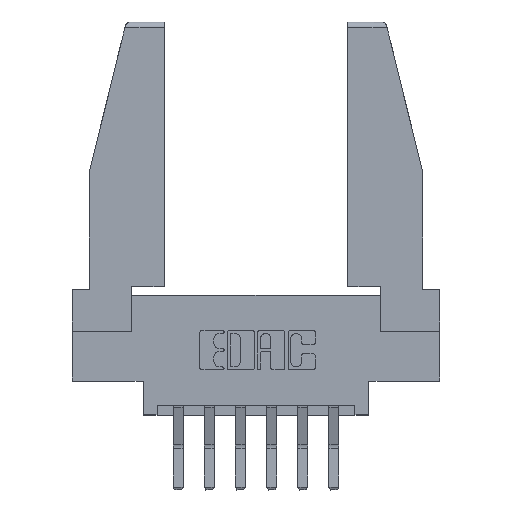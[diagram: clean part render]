
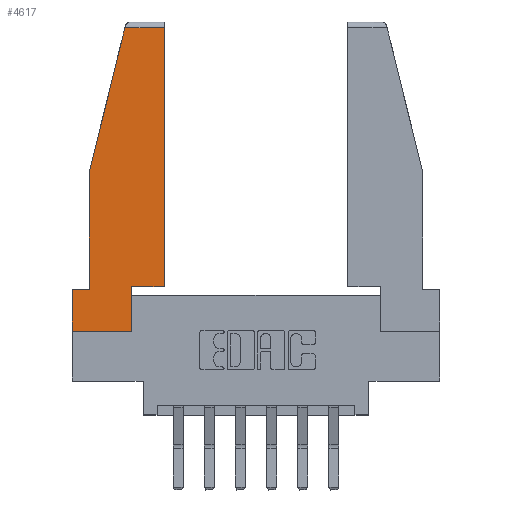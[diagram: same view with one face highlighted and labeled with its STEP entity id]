
A CAD part, top view. The second image highlights one B-rep face of the part: STEP entity #4617.
In plain terms, the highlighted planar face has unit normal (0, 0, 1).
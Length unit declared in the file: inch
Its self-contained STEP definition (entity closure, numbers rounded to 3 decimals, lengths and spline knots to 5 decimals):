
#335 = FACE_OUTER_BOUND ( 'NONE', #1896, .T. ) ;
#481 = ORIENTED_EDGE ( 'NONE', *, *, #3997, .T. ) ;
#562 = VERTEX_POINT ( 'NONE', #1322 ) ;
#895 = CARTESIAN_POINT ( 'NONE',  ( 0.461, 1.52, 0. ) ) ;
#1084 = VERTEX_POINT ( 'NONE', #895 ) ;
#1322 = CARTESIAN_POINT ( 'NONE',  ( 0.297, 0.223, 0. ) ) ;
#1429 = LINE ( 'NONE', #7265, #10963 ) ;
#1442 = CARTESIAN_POINT ( 'NONE',  ( 0.297, 0.223, 0. ) ) ;
#1462 = CARTESIAN_POINT ( 'NONE',  ( 0.086, 0.8, 0. ) ) ;
#1509 = VERTEX_POINT ( 'NONE', #9792 ) ;
#1642 = CARTESIAN_POINT ( 'NONE',  ( 0., 1.52, 0. ) ) ;
#1672 = VERTEX_POINT ( 'NONE', #10440 ) ;
#1715 = LINE ( 'NONE', #9343, #6177 ) ;
#1764 = DIRECTION ( 'NONE',  ( 0., 1., 0. ) ) ;
#1896 = EDGE_LOOP ( 'NONE', ( #10726, #5949, #8733, #7139, #9269, #3287, #5009, #481, #10562 ) ) ;
#2374 = VERTEX_POINT ( 'NONE', #8018 ) ;
#2620 = DIRECTION ( 'NONE',  ( 1., 0., 0. ) ) ;
#2673 = CARTESIAN_POINT ( 'NONE',  ( 0.086, 0.21, 0. ) ) ;
#2810 = CARTESIAN_POINT ( 'NONE',  ( 0.297, 0., 0. ) ) ;
#3060 = CARTESIAN_POINT ( 'NONE',  ( 0.2636, 1.52, 0. ) ) ;
#3287 = ORIENTED_EDGE ( 'NONE', *, *, #10573, .T. ) ;
#3321 = LINE ( 'NONE', #1642, #5349 ) ;
#3375 = CARTESIAN_POINT ( 'NONE',  ( 0.271, 1.55, 0. ) ) ;
#3633 = LINE ( 'NONE', #5037, #11858 ) ;
#3917 = DIRECTION ( 'NONE',  ( -1., 0., 0. ) ) ;
#3997 = EDGE_CURVE ( 'NONE', #1672, #562, #7844, .T. ) ;
#4175 = LINE ( 'NONE', #9431, #11834 ) ;
#4617 = ADVANCED_FACE ( 'NONE', ( #335 ), #5461, .T. ) ;
#5009 = ORIENTED_EDGE ( 'NONE', *, *, #9911, .T. ) ;
#5037 = CARTESIAN_POINT ( 'NONE',  ( 0.461, 0.223, 0. ) ) ;
#5315 = VECTOR ( 'NONE', #5523, 39.37008 ) ;
#5349 = VECTOR ( 'NONE', #7009, 39.37008 ) ;
#5395 = VECTOR ( 'NONE', #1764, 39.37008 ) ;
#5461 = PLANE ( 'NONE',  #7144 ) ;
#5523 = DIRECTION ( 'NONE',  ( 0., -1., 0. ) ) ;
#5735 = LINE ( 'NONE', #1442, #11045 ) ;
#5809 = VERTEX_POINT ( 'NONE', #1462 ) ;
#5937 = EDGE_CURVE ( 'NONE', #10702, #5809, #10527, .T. ) ;
#5949 = ORIENTED_EDGE ( 'NONE', *, *, #9807, .T. ) ;
#6177 = VECTOR ( 'NONE', #9271, 39.37008 ) ;
#6497 = CARTESIAN_POINT ( 'NONE',  ( 0., 0.21, 0. ) ) ;
#6789 = VERTEX_POINT ( 'NONE', #2673 ) ;
#6962 = EDGE_CURVE ( 'NONE', #5809, #6789, #8760, .T. ) ;
#7009 = DIRECTION ( 'NONE',  ( -1., 0., 0. ) ) ;
#7139 = ORIENTED_EDGE ( 'NONE', *, *, #6962, .T. ) ;
#7144 = AXIS2_PLACEMENT_3D ( 'NONE', #8323, #7322, #2620 ) ;
#7265 = CARTESIAN_POINT ( 'NONE',  ( 0., 0., 0. ) ) ;
#7322 = DIRECTION ( 'NONE',  ( 0., 0., 1. ) ) ;
#7844 = LINE ( 'NONE', #2810, #5395 ) ;
#7866 = DIRECTION ( 'NONE',  ( 1., 0., 0. ) ) ;
#8018 = CARTESIAN_POINT ( 'NONE',  ( 0., 0., 0. ) ) ;
#8041 = DIRECTION ( 'NONE',  ( -0.239, -0.971, 0. ) ) ;
#8199 = DIRECTION ( 'NONE',  ( 1., 0., 0. ) ) ;
#8323 = CARTESIAN_POINT ( 'NONE',  ( 0., 0., 0. ) ) ;
#8427 = CARTESIAN_POINT ( 'NONE',  ( 0.086, 0.8, 0. ) ) ;
#8733 = ORIENTED_EDGE ( 'NONE', *, *, #5937, .T. ) ;
#8760 = LINE ( 'NONE', #8427, #5315 ) ;
#9269 = ORIENTED_EDGE ( 'NONE', *, *, #9946, .T. ) ;
#9271 = DIRECTION ( 'NONE',  ( 0., -1., 0. ) ) ;
#9273 = EDGE_CURVE ( 'NONE', #1509, #1084, #3633, .T. ) ;
#9343 = CARTESIAN_POINT ( 'NONE',  ( 0., 0.21, 0. ) ) ;
#9431 = CARTESIAN_POINT ( 'NONE',  ( 0., 0.21, 0. ) ) ;
#9792 = CARTESIAN_POINT ( 'NONE',  ( 0.461, 0.223, 0. ) ) ;
#9807 = EDGE_CURVE ( 'NONE', #1084, #10702, #3321, .T. ) ;
#9911 = EDGE_CURVE ( 'NONE', #2374, #1672, #1429, .T. ) ;
#9946 = EDGE_CURVE ( 'NONE', #6789, #11401, #4175, .T. ) ;
#10440 = CARTESIAN_POINT ( 'NONE',  ( 0.297, 0., 0. ) ) ;
#10527 = LINE ( 'NONE', #3375, #11991 ) ;
#10562 = ORIENTED_EDGE ( 'NONE', *, *, #11865, .T. ) ;
#10573 = EDGE_CURVE ( 'NONE', #11401, #2374, #1715, .T. ) ;
#10610 = DIRECTION ( 'NONE',  ( 0., 1., 0. ) ) ;
#10702 = VERTEX_POINT ( 'NONE', #3060 ) ;
#10726 = ORIENTED_EDGE ( 'NONE', *, *, #9273, .T. ) ;
#10963 = VECTOR ( 'NONE', #8199, 39.37008 ) ;
#11045 = VECTOR ( 'NONE', #7866, 39.37008 ) ;
#11401 = VERTEX_POINT ( 'NONE', #6497 ) ;
#11834 = VECTOR ( 'NONE', #3917, 39.37008 ) ;
#11858 = VECTOR ( 'NONE', #10610, 39.37008 ) ;
#11865 = EDGE_CURVE ( 'NONE', #562, #1509, #5735, .T. ) ;
#11991 = VECTOR ( 'NONE', #8041, 39.37008 ) ;
